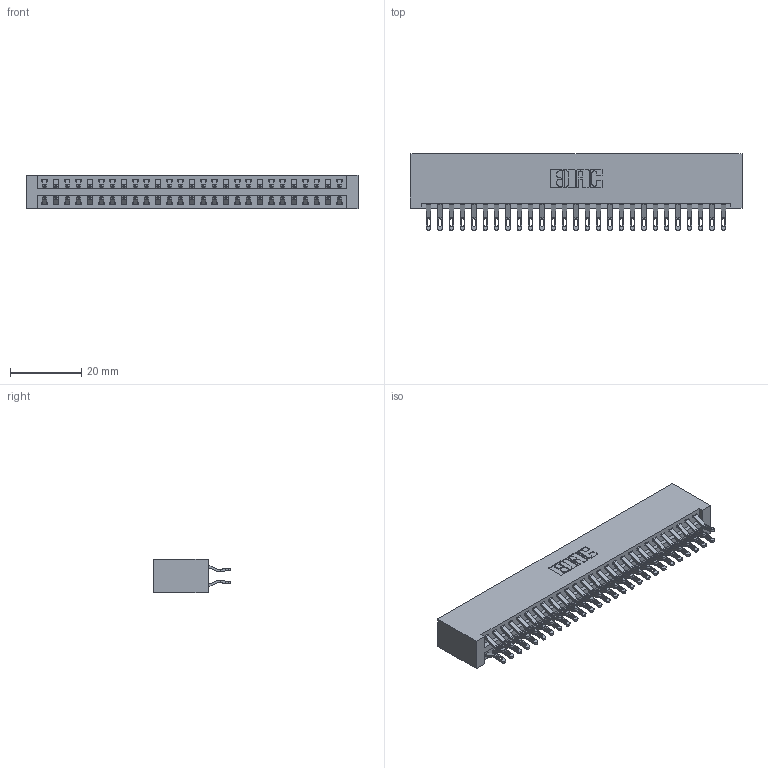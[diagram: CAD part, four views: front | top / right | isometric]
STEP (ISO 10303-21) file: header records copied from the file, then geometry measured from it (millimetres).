
FILE_DESCRIPTION (( 'STEP AP203' ), '1' );
FILE_NAME ('346-054-555-201.STEP', '2022-05-21T03:46:24', ( '' ), ( '' ), 'SwSTEP 2.0', 'SolidWorks 2020', '' );
FILE_SCHEMA (( 'CONFIG_CONTROL_DESIGN' ));
Length unit declared in the file: inch
Products named in the file (3): 345-292-001_555 Tail; 346-054-555-201; 346 Part_No Mounting Lugs
Assembly tree (55 placements, depth 2):
  346-054-555-201
    346 Part_No Mounting Lugs
    345-292-001_555 Tail  x54
Bounding box: 92.96 x 21.46 x 9.4 mm (x, y, z)
Volume: 9678.6 mm3; surface area: 13789.6 mm2
Topology: 55 solids, 55 shells, 3246 faces, 10187 edges, 6790 vertices
Faces by surface type: plane 1854, cylinder 1392
Entity records: 19689 total; most frequent: CARTESIAN_POINT 3298, ORIENTED_EDGE 3202, DIRECTION 2921, EDGE_CURVE 1601, LINE 1349, VECTOR 1349, VERTEX_POINT 1066, AXIS2_PLACEMENT_3D 786
